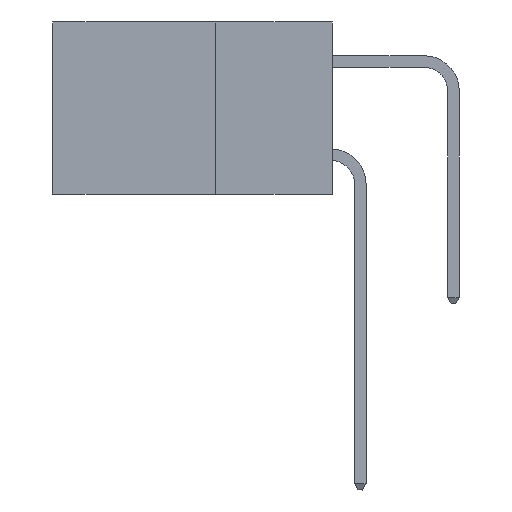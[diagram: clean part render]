
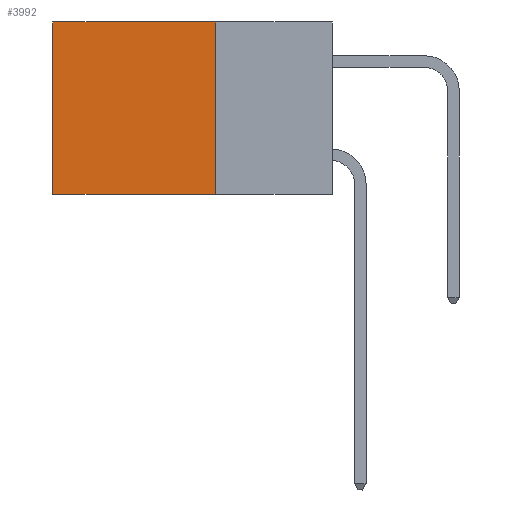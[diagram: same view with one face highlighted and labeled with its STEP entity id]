
A CAD part, left-side view. The second image highlights one B-rep face of the part: STEP entity #3992.
In plain terms, the highlighted planar face has unit normal (-1, 0, 0).
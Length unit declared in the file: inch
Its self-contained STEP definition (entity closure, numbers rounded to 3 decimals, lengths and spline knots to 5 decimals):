
#57 = DIRECTION ( 'NONE',  ( 0., 0., -1. ) ) ;
#394 = VERTEX_POINT ( 'NONE', #9878 ) ;
#1691 = EDGE_LOOP ( 'NONE', ( #13422, #13510, #7926, #8083 ) ) ;
#1741 = DIRECTION ( 'NONE',  ( 0., 0., -1. ) ) ;
#2228 = DIRECTION ( 'NONE',  ( 0., 1., 0. ) ) ;
#2413 = CARTESIAN_POINT ( 'NONE',  ( 0.298, 0.6, -0.37 ) ) ;
#3621 = LINE ( 'NONE', #10796, #4247 ) ;
#3910 = LINE ( 'NONE', #11579, #6744 ) ;
#3992 = ADVANCED_FACE ( 'NONE', ( #15300 ), #9637, .F. ) ;
#4247 = VECTOR ( 'NONE', #1741, 39.37008 ) ;
#4555 = VERTEX_POINT ( 'NONE', #2413 ) ;
#4830 = CARTESIAN_POINT ( 'NONE',  ( 0.298, 0.6, 0. ) ) ;
#5556 = CARTESIAN_POINT ( 'NONE',  ( 0.298, 0.25, -0.37 ) ) ;
#5873 = EDGE_CURVE ( 'NONE', #12870, #4555, #3621, .T. ) ;
#6744 = VECTOR ( 'NONE', #14318, 39.37008 ) ;
#7926 = ORIENTED_EDGE ( 'NONE', *, *, #13927, .F. ) ;
#8083 = ORIENTED_EDGE ( 'NONE', *, *, #15116, .T. ) ;
#8357 = DIRECTION ( 'NONE',  ( 0., 0., -1. ) ) ;
#8583 = LINE ( 'NONE', #10038, #15508 ) ;
#8617 = VERTEX_POINT ( 'NONE', #5556 ) ;
#9637 = PLANE ( 'NONE',  #15975 ) ;
#9878 = CARTESIAN_POINT ( 'NONE',  ( 0.298, 0.25, 0. ) ) ;
#10038 = CARTESIAN_POINT ( 'NONE',  ( 0.298, 0.25, -0.37 ) ) ;
#10796 = CARTESIAN_POINT ( 'NONE',  ( 0.298, 0.6, 0. ) ) ;
#10945 = DIRECTION ( 'NONE',  ( 1., 0., 0. ) ) ;
#11579 = CARTESIAN_POINT ( 'NONE',  ( 0.298, 0.25, 0. ) ) ;
#12108 = VECTOR ( 'NONE', #57, 39.37008 ) ;
#12870 = VERTEX_POINT ( 'NONE', #4830 ) ;
#12941 = EDGE_CURVE ( 'NONE', #8617, #4555, #8583, .T. ) ;
#13422 = ORIENTED_EDGE ( 'NONE', *, *, #5873, .T. ) ;
#13510 = ORIENTED_EDGE ( 'NONE', *, *, #12941, .F. ) ;
#13927 = EDGE_CURVE ( 'NONE', #394, #8617, #14762, .T. ) ;
#14318 = DIRECTION ( 'NONE',  ( 0., 1., 0. ) ) ;
#14762 = LINE ( 'NONE', #16906, #12108 ) ;
#15116 = EDGE_CURVE ( 'NONE', #394, #12870, #3910, .T. ) ;
#15300 = FACE_OUTER_BOUND ( 'NONE', #1691, .T. ) ;
#15508 = VECTOR ( 'NONE', #2228, 39.37008 ) ;
#15975 = AXIS2_PLACEMENT_3D ( 'NONE', #16227, #10945, #8357 ) ;
#16227 = CARTESIAN_POINT ( 'NONE',  ( 0.298, 0.25, 0. ) ) ;
#16906 = CARTESIAN_POINT ( 'NONE',  ( 0.298, 0.25, 0. ) ) ;
